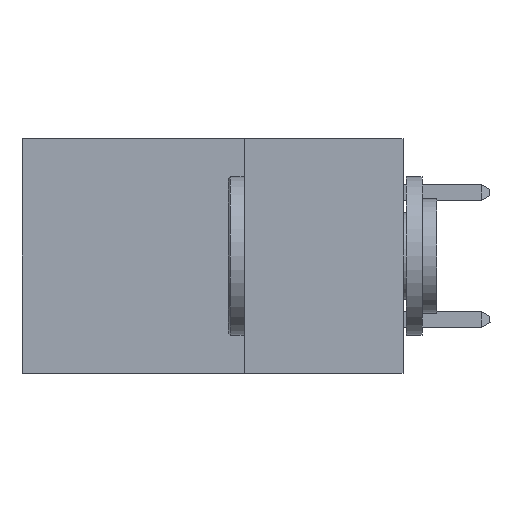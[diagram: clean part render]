
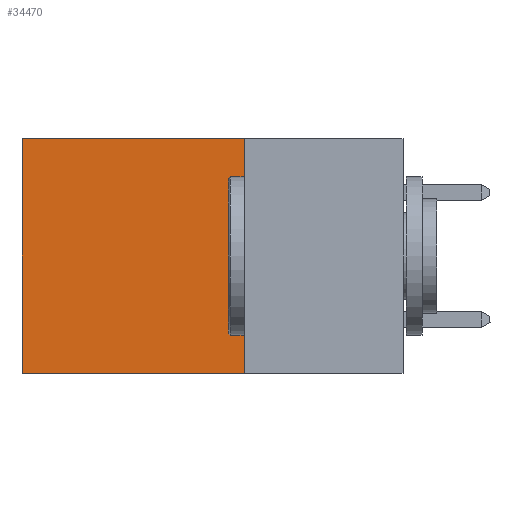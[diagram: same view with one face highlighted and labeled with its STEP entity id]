
A CAD part, left-side view. The second image highlights one B-rep face of the part: STEP entity #34470.
In plain terms, the highlighted planar face has unit normal (-1, 0, 0).
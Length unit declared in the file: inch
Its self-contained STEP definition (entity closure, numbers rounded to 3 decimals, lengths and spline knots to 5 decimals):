
#777 = EDGE_CURVE ( 'NONE', #19421, #34548, #20993, .T. ) ;
#853 = ORIENTED_EDGE ( 'NONE', *, *, #777, .F. ) ;
#1811 = PLANE ( 'NONE',  #10038 ) ;
#2236 = DIRECTION ( 'NONE',  ( 0., 0., -1. ) ) ;
#6719 = VERTEX_POINT ( 'NONE', #24438 ) ;
#7229 = DIRECTION ( 'NONE',  ( 0., 1., 0. ) ) ;
#8520 = EDGE_CURVE ( 'NONE', #6719, #22158, #40340, .T. ) ;
#8749 = CARTESIAN_POINT ( 'NONE',  ( 0.2875, 0.25, 0. ) ) ;
#10038 = AXIS2_PLACEMENT_3D ( 'NONE', #8749, #34933, #2236 ) ;
#11662 = LINE ( 'NONE', #36747, #36878 ) ;
#12343 = CARTESIAN_POINT ( 'NONE',  ( 0.2875, 0.25, -0.37 ) ) ;
#14410 = CARTESIAN_POINT ( 'NONE',  ( 0.2875, 0.25, 0. ) ) ;
#14730 = CARTESIAN_POINT ( 'NONE',  ( 0.2875, 0.25, -0.37 ) ) ;
#16009 = CARTESIAN_POINT ( 'NONE',  ( 0.2875, 0.6, 0. ) ) ;
#19421 = VERTEX_POINT ( 'NONE', #14410 ) ;
#19913 = ORIENTED_EDGE ( 'NONE', *, *, #38128, .T. ) ;
#20993 = LINE ( 'NONE', #34540, #29223 ) ;
#22158 = VERTEX_POINT ( 'NONE', #35522 ) ;
#22493 = DIRECTION ( 'NONE',  ( 0., 0., -1. ) ) ;
#23807 = EDGE_CURVE ( 'NONE', #34548, #22158, #36045, .T. ) ;
#24438 = CARTESIAN_POINT ( 'NONE',  ( 0.2875, 0.6, 0. ) ) ;
#27289 = VECTOR ( 'NONE', #27690, 39.37008 ) ;
#27413 = VECTOR ( 'NONE', #22493, 39.37008 ) ;
#27690 = DIRECTION ( 'NONE',  ( 0., 1., 0. ) ) ;
#27891 = ORIENTED_EDGE ( 'NONE', *, *, #23807, .F. ) ;
#29223 = VECTOR ( 'NONE', #40782, 39.37008 ) ;
#30543 = FACE_OUTER_BOUND ( 'NONE', #42155, .T. ) ;
#34470 = ADVANCED_FACE ( 'NONE', ( #30543 ), #1811, .F. ) ;
#34540 = CARTESIAN_POINT ( 'NONE',  ( 0.2875, 0.25, 0. ) ) ;
#34548 = VERTEX_POINT ( 'NONE', #12343 ) ;
#34933 = DIRECTION ( 'NONE',  ( 1., 0., 0. ) ) ;
#35522 = CARTESIAN_POINT ( 'NONE',  ( 0.2875, 0.6, -0.37 ) ) ;
#36045 = LINE ( 'NONE', #14730, #27289 ) ;
#36747 = CARTESIAN_POINT ( 'NONE',  ( 0.2875, 0.25, 0. ) ) ;
#36878 = VECTOR ( 'NONE', #7229, 39.37008 ) ;
#38128 = EDGE_CURVE ( 'NONE', #19421, #6719, #11662, .T. ) ;
#39616 = ORIENTED_EDGE ( 'NONE', *, *, #8520, .T. ) ;
#40340 = LINE ( 'NONE', #16009, #27413 ) ;
#40782 = DIRECTION ( 'NONE',  ( 0., 0., -1. ) ) ;
#42155 = EDGE_LOOP ( 'NONE', ( #39616, #27891, #853, #19913 ) ) ;
